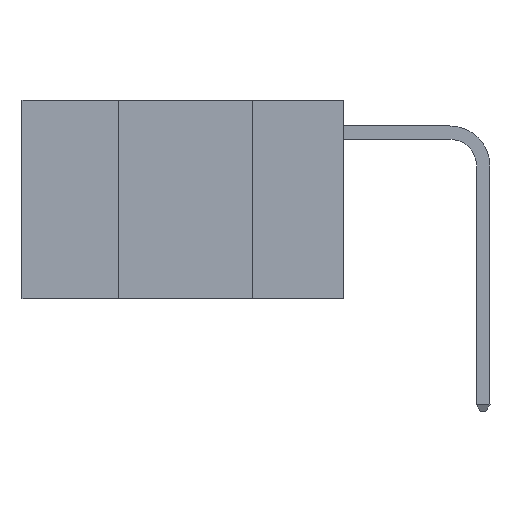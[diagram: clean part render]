
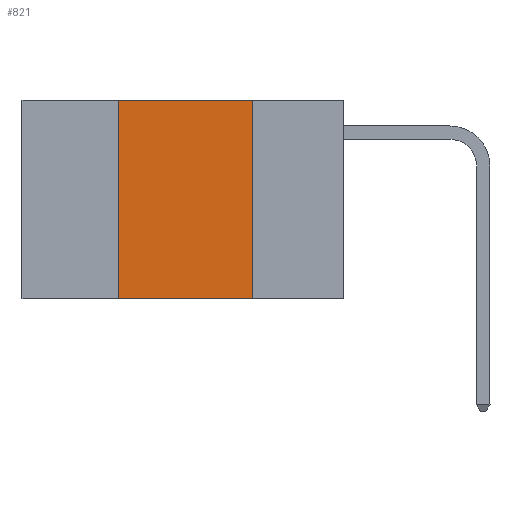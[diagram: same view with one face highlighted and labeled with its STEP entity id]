
A CAD part, left-side view. The second image highlights one B-rep face of the part: STEP entity #821.
In plain terms, the highlighted planar face has unit normal (-1, 0, 0).
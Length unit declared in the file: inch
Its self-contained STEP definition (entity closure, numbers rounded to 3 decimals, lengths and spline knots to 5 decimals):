
#513 = VERTEX_POINT ( 'NONE', #22406 ) ;
#821 = ADVANCED_FACE ( 'NONE', ( #19309 ), #18711, .F. ) ;
#1999 = CARTESIAN_POINT ( 'NONE',  ( 0., 0.42, -0.37 ) ) ;
#2828 = LINE ( 'NONE', #6583, #4908 ) ;
#2910 = LINE ( 'NONE', #21861, #17223 ) ;
#4036 = EDGE_LOOP ( 'NONE', ( #7233, #9043, #9598, #12761 ) ) ;
#4556 = VERTEX_POINT ( 'NONE', #22509 ) ;
#4908 = VECTOR ( 'NONE', #21207, 39.37008 ) ;
#6583 = CARTESIAN_POINT ( 'NONE',  ( 0., 0.6, 0. ) ) ;
#7233 = ORIENTED_EDGE ( 'NONE', *, *, #7257, .F. ) ;
#7257 = EDGE_CURVE ( 'NONE', #4556, #513, #2910, .T. ) ;
#7276 = LINE ( 'NONE', #11464, #16538 ) ;
#7451 = DIRECTION ( 'NONE',  ( 0., 0., 1. ) ) ;
#8762 = EDGE_CURVE ( 'NONE', #11860, #18471, #14640, .T. ) ;
#9043 = ORIENTED_EDGE ( 'NONE', *, *, #19189, .F. ) ;
#9317 = CARTESIAN_POINT ( 'NONE',  ( 0., 0.42, 0. ) ) ;
#9598 = ORIENTED_EDGE ( 'NONE', *, *, #8762, .F. ) ;
#11464 = CARTESIAN_POINT ( 'NONE',  ( 0., 0.6, -0.37 ) ) ;
#11860 = VERTEX_POINT ( 'NONE', #1999 ) ;
#12761 = ORIENTED_EDGE ( 'NONE', *, *, #19978, .T. ) ;
#13332 = DIRECTION ( 'NONE',  ( 0., -1., 0. ) ) ;
#14640 = LINE ( 'NONE', #9317, #18299 ) ;
#16538 = VECTOR ( 'NONE', #13332, 39.37008 ) ;
#17223 = VECTOR ( 'NONE', #23612, 39.37008 ) ;
#18299 = VECTOR ( 'NONE', #7451, 39.37008 ) ;
#18471 = VERTEX_POINT ( 'NONE', #22359 ) ;
#18564 = DIRECTION ( 'NONE',  ( 0., 0., -1. ) ) ;
#18570 = DIRECTION ( 'NONE',  ( 1., 0., 0. ) ) ;
#18711 = PLANE ( 'NONE',  #22713 ) ;
#18831 = CARTESIAN_POINT ( 'NONE',  ( 0., 0.6, 0. ) ) ;
#19189 = EDGE_CURVE ( 'NONE', #18471, #4556, #2828, .T. ) ;
#19309 = FACE_OUTER_BOUND ( 'NONE', #4036, .T. ) ;
#19978 = EDGE_CURVE ( 'NONE', #11860, #513, #7276, .T. ) ;
#21207 = DIRECTION ( 'NONE',  ( 0., -1., 0. ) ) ;
#21861 = CARTESIAN_POINT ( 'NONE',  ( 0., 0.17, 0. ) ) ;
#22359 = CARTESIAN_POINT ( 'NONE',  ( 0., 0.42, 0. ) ) ;
#22406 = CARTESIAN_POINT ( 'NONE',  ( 0., 0.17, -0.37 ) ) ;
#22509 = CARTESIAN_POINT ( 'NONE',  ( 0., 0.17, 0. ) ) ;
#22713 = AXIS2_PLACEMENT_3D ( 'NONE', #18831, #18570, #18564 ) ;
#23612 = DIRECTION ( 'NONE',  ( 0., 0., -1. ) ) ;
